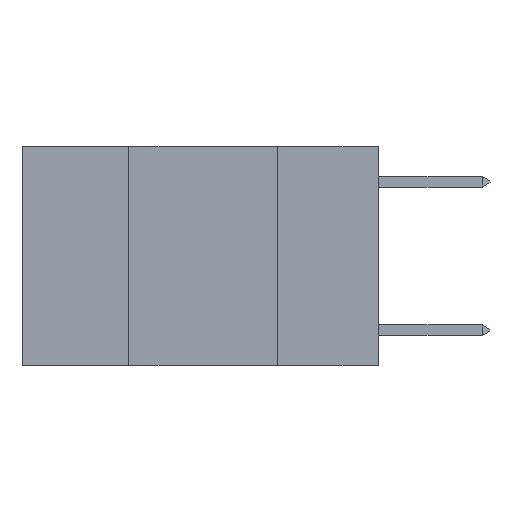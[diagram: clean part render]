
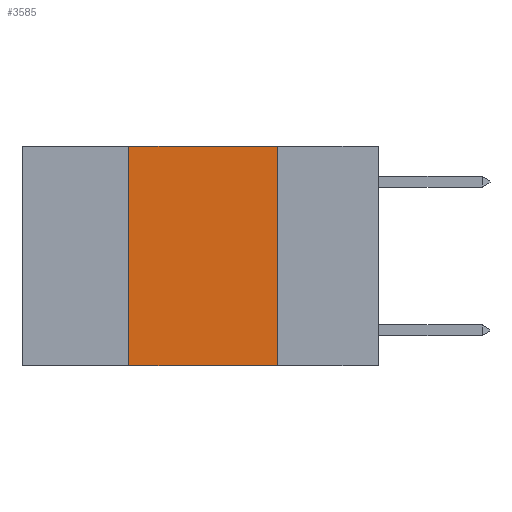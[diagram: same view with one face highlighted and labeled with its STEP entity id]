
A CAD part, left-side view. The second image highlights one B-rep face of the part: STEP entity #3585.
In plain terms, the highlighted planar face has unit normal (-1, 0, 0).
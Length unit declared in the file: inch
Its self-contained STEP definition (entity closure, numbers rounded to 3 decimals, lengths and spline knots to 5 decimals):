
#99 = CARTESIAN_POINT ( 'NONE',  ( 0., 0.6, -0.37 ) ) ;
#252 = LINE ( 'NONE', #99, #14634 ) ;
#614 = EDGE_LOOP ( 'NONE', ( #1166, #7573, #1400, #1621 ) ) ;
#634 = PLANE ( 'NONE',  #16848 ) ;
#767 = CARTESIAN_POINT ( 'NONE',  ( 0., 0.42, 0. ) ) ;
#1166 = ORIENTED_EDGE ( 'NONE', *, *, #10339, .F. ) ;
#1400 = ORIENTED_EDGE ( 'NONE', *, *, #11178, .F. ) ;
#1621 = ORIENTED_EDGE ( 'NONE', *, *, #12956, .T. ) ;
#2816 = DIRECTION ( 'NONE',  ( 0., 0., -1. ) ) ;
#3239 = CARTESIAN_POINT ( 'NONE',  ( 0., 0.42, 0. ) ) ;
#3585 = ADVANCED_FACE ( 'NONE', ( #11066 ), #634, .F. ) ;
#4040 = CARTESIAN_POINT ( 'NONE',  ( 0., 0.17, -0.37 ) ) ;
#5081 = CARTESIAN_POINT ( 'NONE',  ( 0., 0.6, 0. ) ) ;
#6072 = LINE ( 'NONE', #5081, #13390 ) ;
#6371 = DIRECTION ( 'NONE',  ( 0., 0., -1. ) ) ;
#7549 = DIRECTION ( 'NONE',  ( 0., 0., 1. ) ) ;
#7573 = ORIENTED_EDGE ( 'NONE', *, *, #12582, .F. ) ;
#7800 = CARTESIAN_POINT ( 'NONE',  ( 0., 0.17, 0. ) ) ;
#7873 = VECTOR ( 'NONE', #2816, 39.37008 ) ;
#8920 = VERTEX_POINT ( 'NONE', #4040 ) ;
#9128 = LINE ( 'NONE', #3239, #12380 ) ;
#9852 = CARTESIAN_POINT ( 'NONE',  ( 0., 0.17, 0. ) ) ;
#9999 = VERTEX_POINT ( 'NONE', #7800 ) ;
#10006 = CARTESIAN_POINT ( 'NONE',  ( 0., 0.42, -0.37 ) ) ;
#10339 = EDGE_CURVE ( 'NONE', #9999, #8920, #15519, .T. ) ;
#11066 = FACE_OUTER_BOUND ( 'NONE', #614, .T. ) ;
#11178 = EDGE_CURVE ( 'NONE', #17833, #13265, #9128, .T. ) ;
#12380 = VECTOR ( 'NONE', #7549, 39.37008 ) ;
#12582 = EDGE_CURVE ( 'NONE', #13265, #9999, #6072, .T. ) ;
#12956 = EDGE_CURVE ( 'NONE', #17833, #8920, #252, .T. ) ;
#13233 = CARTESIAN_POINT ( 'NONE',  ( 0., 0.6, 0. ) ) ;
#13265 = VERTEX_POINT ( 'NONE', #767 ) ;
#13390 = VECTOR ( 'NONE', #14727, 39.37008 ) ;
#14575 = DIRECTION ( 'NONE',  ( 1., 0., 0. ) ) ;
#14634 = VECTOR ( 'NONE', #16649, 39.37008 ) ;
#14727 = DIRECTION ( 'NONE',  ( 0., -1., 0. ) ) ;
#15519 = LINE ( 'NONE', #9852, #7873 ) ;
#16649 = DIRECTION ( 'NONE',  ( 0., -1., 0. ) ) ;
#16848 = AXIS2_PLACEMENT_3D ( 'NONE', #13233, #14575, #6371 ) ;
#17833 = VERTEX_POINT ( 'NONE', #10006 ) ;
